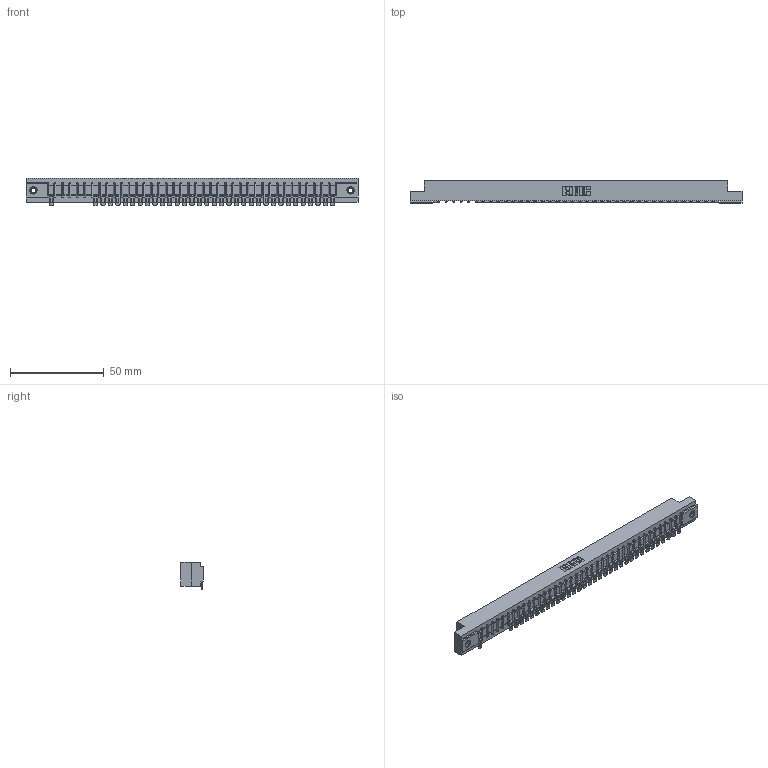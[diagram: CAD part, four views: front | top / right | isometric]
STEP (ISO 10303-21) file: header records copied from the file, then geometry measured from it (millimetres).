
FILE_DESCRIPTION (( 'STEP AP203' ), '1' );
FILE_NAME ('357-039-554-107.STEP', '2018-08-11T04:29:42', ( '' ), ( '' ), 'SwSTEP 2.0', 'SolidWorks 2016', '' );
FILE_SCHEMA (( 'CONFIG_CONTROL_DESIGN' ));
Length unit declared in the file: inch
Products named in the file (4): 307 Part_.156 Dia Mounting Holes; 307-290-002_554; 345-250-001_345-250-005-103; 357-039-554-107
Assembly tree (37 placements, depth 2):
  357-039-554-107
    307 Part_.156 Dia Mounting Holes
    307-290-002_554  x34
    345-250-001_345-250-005-103  x2
Bounding box: 177.55 x 12.01 x 14.52 mm (x, y, z)
Volume: 18831.3 mm3; surface area: 22848.7 mm2
Topology: 37 solids, 37 shells, 3072 faces, 9381 edges, 6138 vertices
Faces by surface type: plane 1726, cylinder 1250, sphere 80, cone 12, torus 4
Entity records: 35794 total; most frequent: CARTESIAN_POINT 6040, ORIENTED_EDGE 6028, DIRECTION 5880, EDGE_CURVE 3014, VECTOR 2300, LINE 2300, VERTEX_POINT 1950, AXIS2_PLACEMENT_3D 1790
